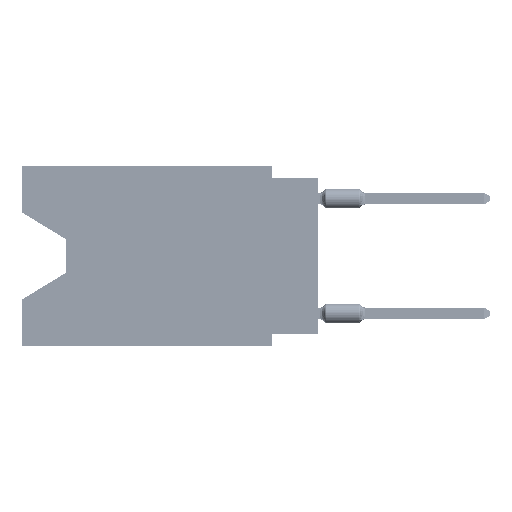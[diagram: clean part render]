
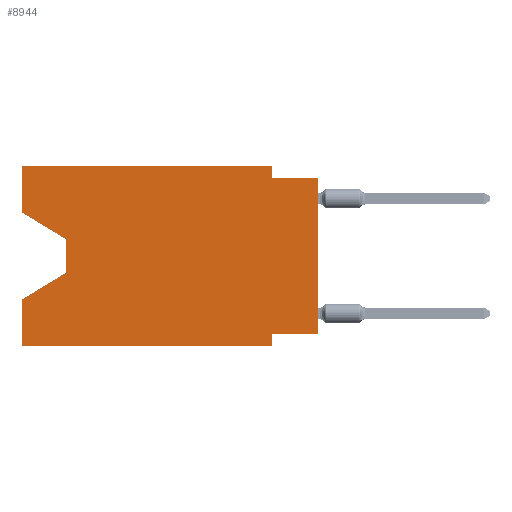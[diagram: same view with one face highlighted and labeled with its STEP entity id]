
A CAD part, left-side view. The second image highlights one B-rep face of the part: STEP entity #8944.
In plain terms, the highlighted planar face has unit normal (-1, 0, 0).
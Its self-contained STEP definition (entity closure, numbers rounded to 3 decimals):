
#1203 = DIRECTION ( 'NONE',  ( 0., 0., -1. ) ) ;
#1610 = DIRECTION ( 'NONE',  ( 0., 0., 1. ) ) ;
#2081 = VERTEX_POINT ( 'NONE', #69920 ) ;
#2200 = CARTESIAN_POINT ( 'NONE',  ( 0., 0., -0.635 ) ) ;
#3395 = CARTESIAN_POINT ( 'NONE',  ( 0., 16.383, -2.546 ) ) ;
#3714 = VECTOR ( 'NONE', #18185, 1000. ) ;
#4135 = LINE ( 'NONE', #18203, #42709 ) ;
#5992 = CARTESIAN_POINT ( 'NONE',  ( 0., 16.383, 0. ) ) ;
#6122 = VECTOR ( 'NONE', #51776, 1000. ) ;
#7541 = VECTOR ( 'NONE', #24067, 1000. ) ;
#8438 = CARTESIAN_POINT ( 'NONE',  ( 0., 16.383, 0. ) ) ;
#8944 = ADVANCED_FACE ( 'NONE', ( #20827 ), #72964, .F. ) ;
#12191 = CARTESIAN_POINT ( 'NONE',  ( 0., 2.54, -9.906 ) ) ;
#12893 = EDGE_LOOP ( 'NONE', ( #42285, #20205, #83236, #68047, #25422, #77479, #60334, #19412, #66581, #51044, #77665, #80240 ) ) ;
#13179 = CARTESIAN_POINT ( 'NONE',  ( 0., 16.383, 0. ) ) ;
#13677 = VERTEX_POINT ( 'NONE', #45134 ) ;
#15370 = VECTOR ( 'NONE', #67479, 1000. ) ;
#18185 = DIRECTION ( 'NONE',  ( 0., 0., -1. ) ) ;
#18203 = CARTESIAN_POINT ( 'NONE',  ( 0., 13.97, -5.893 ) ) ;
#19412 = ORIENTED_EDGE ( 'NONE', *, *, #21708, .T. ) ;
#20205 = ORIENTED_EDGE ( 'NONE', *, *, #53239, .T. ) ;
#20422 = VECTOR ( 'NONE', #52526, 1000. ) ;
#20528 = LINE ( 'NONE', #60668, #27097 ) ;
#20827 = FACE_OUTER_BOUND ( 'NONE', #12893, .T. ) ;
#21708 = EDGE_CURVE ( 'NONE', #13677, #25396, #76995, .T. ) ;
#22526 = VECTOR ( 'NONE', #25140, 1000. ) ;
#24067 = DIRECTION ( 'NONE',  ( 0., 0., 1. ) ) ;
#24195 = CARTESIAN_POINT ( 'NONE',  ( 0., 2.54, -9.906 ) ) ;
#24397 = LINE ( 'NONE', #5992, #81475 ) ;
#25140 = DIRECTION ( 'NONE',  ( 0., -1., 0. ) ) ;
#25213 = LINE ( 'NONE', #57687, #20422 ) ;
#25396 = VERTEX_POINT ( 'NONE', #2200 ) ;
#25422 = ORIENTED_EDGE ( 'NONE', *, *, #33245, .T. ) ;
#27097 = VECTOR ( 'NONE', #53434, 1000. ) ;
#29511 = VERTEX_POINT ( 'NONE', #32327 ) ;
#29733 = VERTEX_POINT ( 'NONE', #75394 ) ;
#30479 = LINE ( 'NONE', #56535, #7541 ) ;
#31033 = LINE ( 'NONE', #24195, #3714 ) ;
#31151 = LINE ( 'NONE', #76431, #22526 ) ;
#32327 = CARTESIAN_POINT ( 'NONE',  ( 0., 2.54, -9.271 ) ) ;
#33245 = EDGE_CURVE ( 'NONE', #53966, #36619, #31151, .T. ) ;
#34130 = LINE ( 'NONE', #66154, #62796 ) ;
#36619 = VERTEX_POINT ( 'NONE', #12191 ) ;
#38785 = EDGE_CURVE ( 'NONE', #29733, #54594, #24397, .T. ) ;
#38999 = EDGE_CURVE ( 'NONE', #29511, #36619, #31033, .T. ) ;
#39552 = AXIS2_PLACEMENT_3D ( 'NONE', #13179, #66979, #1203 ) ;
#40541 = DIRECTION ( 'NONE',  ( 0., -1., 0. ) ) ;
#41027 = LINE ( 'NONE', #3395, #15370 ) ;
#41132 = LINE ( 'NONE', #60745, #64914 ) ;
#41550 = DIRECTION ( 'NONE',  ( 0., 0., -1. ) ) ;
#42285 = ORIENTED_EDGE ( 'NONE', *, *, #45006, .T. ) ;
#42709 = VECTOR ( 'NONE', #43867, 1000. ) ;
#43867 = DIRECTION ( 'NONE',  ( 0., 0.855, -0.519 ) ) ;
#45006 = EDGE_CURVE ( 'NONE', #72541, #54968, #41027, .T. ) ;
#45134 = CARTESIAN_POINT ( 'NONE',  ( 0., 0., -9.271 ) ) ;
#45497 = EDGE_CURVE ( 'NONE', #53966, #2081, #80640, .T. ) ;
#45622 = CARTESIAN_POINT ( 'NONE',  ( 0., 13.97, -4.013 ) ) ;
#50338 = EDGE_CURVE ( 'NONE', #13677, #29511, #20528, .T. ) ;
#51044 = ORIENTED_EDGE ( 'NONE', *, *, #67512, .F. ) ;
#51361 = CARTESIAN_POINT ( 'NONE',  ( 0., 0., 0. ) ) ;
#51776 = DIRECTION ( 'NONE',  ( 0., 0., 1. ) ) ;
#52526 = DIRECTION ( 'NONE',  ( 0., 0., -1. ) ) ;
#53239 = EDGE_CURVE ( 'NONE', #54968, #56479, #25213, .T. ) ;
#53434 = DIRECTION ( 'NONE',  ( 0., 1., 0. ) ) ;
#53966 = VERTEX_POINT ( 'NONE', #62933 ) ;
#54594 = VERTEX_POINT ( 'NONE', #58945 ) ;
#54968 = VERTEX_POINT ( 'NONE', #45622 ) ;
#56479 = VERTEX_POINT ( 'NONE', #64689 ) ;
#56535 = CARTESIAN_POINT ( 'NONE',  ( 0., 16.383, 0. ) ) ;
#57687 = CARTESIAN_POINT ( 'NONE',  ( 0., 13.97, -4.013 ) ) ;
#57767 = VECTOR ( 'NONE', #1610, 1000. ) ;
#58464 = CARTESIAN_POINT ( 'NONE',  ( 0., 2.54, -0.635 ) ) ;
#58945 = CARTESIAN_POINT ( 'NONE',  ( 0., 2.54, 0. ) ) ;
#59988 = VERTEX_POINT ( 'NONE', #58464 ) ;
#60262 = EDGE_CURVE ( 'NONE', #56479, #2081, #4135, .T. ) ;
#60334 = ORIENTED_EDGE ( 'NONE', *, *, #50338, .F. ) ;
#60668 = CARTESIAN_POINT ( 'NONE',  ( 0., 0., -9.271 ) ) ;
#60745 = CARTESIAN_POINT ( 'NONE',  ( 0., 2.54, 0. ) ) ;
#62796 = VECTOR ( 'NONE', #40541, 1000. ) ;
#62933 = CARTESIAN_POINT ( 'NONE',  ( 0., 16.383, -9.906 ) ) ;
#64689 = CARTESIAN_POINT ( 'NONE',  ( 0., 13.97, -5.893 ) ) ;
#64859 = EDGE_CURVE ( 'NONE', #72541, #29733, #30479, .T. ) ;
#64914 = VECTOR ( 'NONE', #41550, 1000. ) ;
#66154 = CARTESIAN_POINT ( 'NONE',  ( 0., 0., -0.635 ) ) ;
#66581 = ORIENTED_EDGE ( 'NONE', *, *, #77827, .F. ) ;
#66979 = DIRECTION ( 'NONE',  ( 1., 0., 0. ) ) ;
#67479 = DIRECTION ( 'NONE',  ( 0., -0.855, -0.519 ) ) ;
#67512 = EDGE_CURVE ( 'NONE', #54594, #59988, #41132, .T. ) ;
#68047 = ORIENTED_EDGE ( 'NONE', *, *, #45497, .F. ) ;
#69920 = CARTESIAN_POINT ( 'NONE',  ( 0., 16.383, -7.36 ) ) ;
#72541 = VERTEX_POINT ( 'NONE', #76977 ) ;
#72964 = PLANE ( 'NONE',  #39552 ) ;
#75394 = CARTESIAN_POINT ( 'NONE',  ( 0., 16.383, 0. ) ) ;
#76431 = CARTESIAN_POINT ( 'NONE',  ( 0., 16.383, -9.906 ) ) ;
#76977 = CARTESIAN_POINT ( 'NONE',  ( 0., 16.383, -2.546 ) ) ;
#76995 = LINE ( 'NONE', #51361, #6122 ) ;
#77479 = ORIENTED_EDGE ( 'NONE', *, *, #38999, .F. ) ;
#77665 = ORIENTED_EDGE ( 'NONE', *, *, #38785, .F. ) ;
#77774 = DIRECTION ( 'NONE',  ( 0., -1., 0. ) ) ;
#77827 = EDGE_CURVE ( 'NONE', #59988, #25396, #34130, .T. ) ;
#80240 = ORIENTED_EDGE ( 'NONE', *, *, #64859, .F. ) ;
#80640 = LINE ( 'NONE', #8438, #57767 ) ;
#81475 = VECTOR ( 'NONE', #77774, 1000. ) ;
#83236 = ORIENTED_EDGE ( 'NONE', *, *, #60262, .T. ) ;
